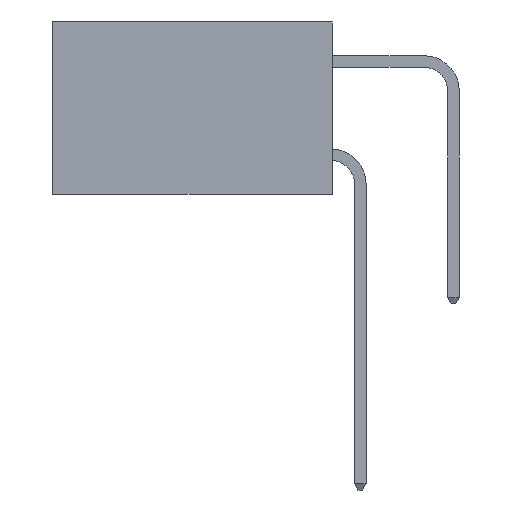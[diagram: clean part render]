
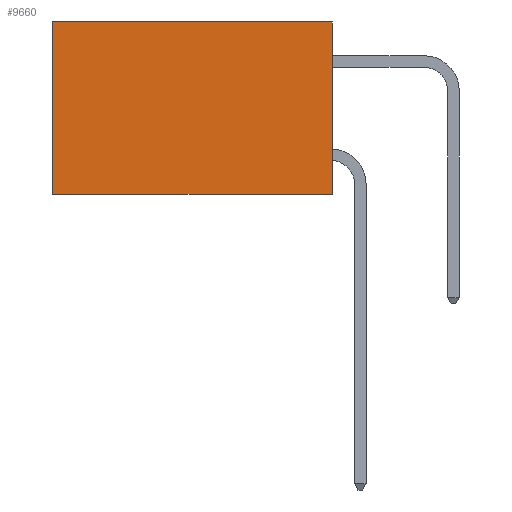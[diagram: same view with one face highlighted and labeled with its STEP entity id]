
A CAD part, left-side view. The second image highlights one B-rep face of the part: STEP entity #9660.
In plain terms, the highlighted planar face has unit normal (-1, 0, 0).
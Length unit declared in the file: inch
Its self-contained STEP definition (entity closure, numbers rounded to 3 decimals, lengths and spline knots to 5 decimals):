
#46 = CARTESIAN_POINT ( 'NONE',  ( 0.2615, 0.6, -0.37 ) ) ;
#99 = EDGE_CURVE ( 'NONE', #8616, #8727, #15811, .T. ) ;
#738 = CARTESIAN_POINT ( 'NONE',  ( 0.2615, 0., -0.37 ) ) ;
#1353 = VECTOR ( 'NONE', #12689, 39.37008 ) ;
#2350 = ORIENTED_EDGE ( 'NONE', *, *, #11102, .F. ) ;
#2456 = VECTOR ( 'NONE', #13067, 39.37008 ) ;
#3772 = AXIS2_PLACEMENT_3D ( 'NONE', #738, #15316, #5739 ) ;
#4645 = ORIENTED_EDGE ( 'NONE', *, *, #12979, .T. ) ;
#4788 = ORIENTED_EDGE ( 'NONE', *, *, #99, .F. ) ;
#5211 = EDGE_LOOP ( 'NONE', ( #16094, #4788, #2350, #4645 ) ) ;
#5674 = PLANE ( 'NONE',  #3772 ) ;
#5739 = DIRECTION ( 'NONE',  ( 0., 0., -1. ) ) ;
#5796 = VECTOR ( 'NONE', #13807, 39.37008 ) ;
#6052 = LINE ( 'NONE', #9743, #18307 ) ;
#7968 = VERTEX_POINT ( 'NONE', #11208 ) ;
#8616 = VERTEX_POINT ( 'NONE', #9585 ) ;
#8727 = VERTEX_POINT ( 'NONE', #46 ) ;
#9585 = CARTESIAN_POINT ( 'NONE',  ( 0.2615, 0., -0.37 ) ) ;
#9660 = ADVANCED_FACE ( 'NONE', ( #20801 ), #5674, .F. ) ;
#9743 = CARTESIAN_POINT ( 'NONE',  ( 0.2615, 0., -0.37 ) ) ;
#10026 = LINE ( 'NONE', #17485, #1353 ) ;
#11102 = EDGE_CURVE ( 'NONE', #19928, #8616, #6052, .T. ) ;
#11208 = CARTESIAN_POINT ( 'NONE',  ( 0.2615, 0.6, 0. ) ) ;
#12118 = CARTESIAN_POINT ( 'NONE',  ( 0.2615, 0.6, -0.37 ) ) ;
#12689 = DIRECTION ( 'NONE',  ( 0., 1., 0. ) ) ;
#12979 = EDGE_CURVE ( 'NONE', #19928, #7968, #10026, .T. ) ;
#13067 = DIRECTION ( 'NONE',  ( 0., 1., 0. ) ) ;
#13807 = DIRECTION ( 'NONE',  ( 0., 0., -1. ) ) ;
#14261 = CARTESIAN_POINT ( 'NONE',  ( 0.2615, 0., 0. ) ) ;
#14335 = LINE ( 'NONE', #12118, #5796 ) ;
#15316 = DIRECTION ( 'NONE',  ( 1., 0., 0. ) ) ;
#15702 = EDGE_CURVE ( 'NONE', #7968, #8727, #14335, .T. ) ;
#15811 = LINE ( 'NONE', #17146, #2456 ) ;
#16065 = DIRECTION ( 'NONE',  ( 0., 0., -1. ) ) ;
#16094 = ORIENTED_EDGE ( 'NONE', *, *, #15702, .T. ) ;
#17146 = CARTESIAN_POINT ( 'NONE',  ( 0.2615, 0., -0.37 ) ) ;
#17485 = CARTESIAN_POINT ( 'NONE',  ( 0.2615, 0., 0. ) ) ;
#18307 = VECTOR ( 'NONE', #16065, 39.37008 ) ;
#19928 = VERTEX_POINT ( 'NONE', #14261 ) ;
#20801 = FACE_OUTER_BOUND ( 'NONE', #5211, .T. ) ;
